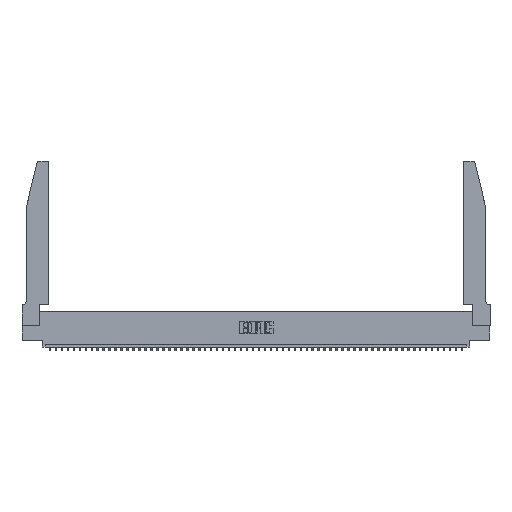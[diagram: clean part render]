
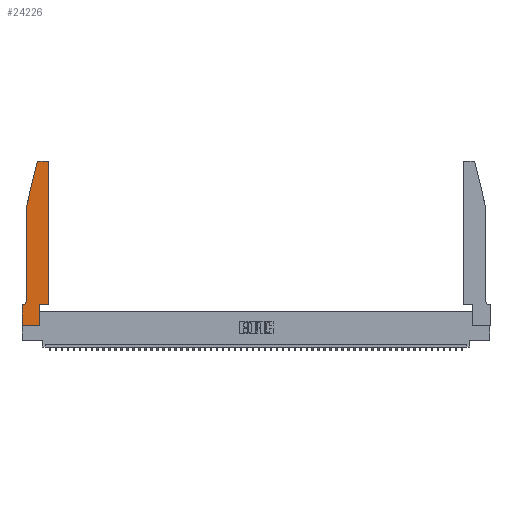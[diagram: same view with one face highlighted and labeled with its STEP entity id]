
A CAD part, top view. The second image highlights one B-rep face of the part: STEP entity #24226.
In plain terms, the highlighted planar face has unit normal (0, 0, 1).
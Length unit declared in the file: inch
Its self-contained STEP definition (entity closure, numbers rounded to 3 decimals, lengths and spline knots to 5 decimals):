
#601 = CARTESIAN_POINT ( 'NONE',  ( 0.284, 2.75, 0.37 ) ) ;
#662 = AXIS2_PLACEMENT_3D ( 'NONE', #33011, #7484, #36627 ) ;
#932 = VERTEX_POINT ( 'NONE', #28533 ) ;
#977 = ORIENTED_EDGE ( 'NONE', *, *, #35297, .T. ) ;
#1527 = CARTESIAN_POINT ( 'NONE',  ( 0.2865, 0.35, 0.37 ) ) ;
#1742 = LINE ( 'NONE', #27572, #7127 ) ;
#2084 = AXIS2_PLACEMENT_3D ( 'NONE', #19080, #23292, #15078 ) ;
#2785 = DIRECTION ( 'NONE',  ( 1., 0., 0. ) ) ;
#3431 = CARTESIAN_POINT ( 'NONE',  ( 0.25487, 2.72718, 0.37 ) ) ;
#3888 = CIRCLE ( 'NONE', #662, 0.03 ) ;
#4181 = AXIS2_PLACEMENT_3D ( 'NONE', #37291, #37455, #8630 ) ;
#4629 = VERTEX_POINT ( 'NONE', #11432 ) ;
#5304 = DIRECTION ( 'NONE',  ( 1., 0., 0. ) ) ;
#5510 = EDGE_CURVE ( 'NONE', #30403, #42698, #13013, .T. ) ;
#5828 = CARTESIAN_POINT ( 'NONE',  ( 0.4205, 2.72, 0.37 ) ) ;
#7127 = VECTOR ( 'NONE', #14575, 39.37008 ) ;
#7484 = DIRECTION ( 'NONE',  ( 0., 0., 1. ) ) ;
#7656 = EDGE_CURVE ( 'NONE', #35112, #29569, #52413, .T. ) ;
#7732 = ORIENTED_EDGE ( 'NONE', *, *, #39719, .T. ) ;
#8617 = DIRECTION ( 'NONE',  ( 0., -1., 0. ) ) ;
#8630 = DIRECTION ( 'NONE',  ( 1., 0., 0. ) ) ;
#9082 = CARTESIAN_POINT ( 'NONE',  ( 0., 0., 0.37 ) ) ;
#9317 = ORIENTED_EDGE ( 'NONE', *, *, #26377, .T. ) ;
#9449 = LINE ( 'NONE', #18105, #13400 ) ;
#11432 = CARTESIAN_POINT ( 'NONE',  ( 0.2865, 0., 0.37 ) ) ;
#11755 = EDGE_LOOP ( 'NONE', ( #43595, #7732, #24595, #18098, #31854, #32771, #25570, #9317, #977, #16857, #46579, #27250 ) ) ;
#11914 = DIRECTION ( 'NONE',  ( 0., 1., 0. ) ) ;
#13013 = LINE ( 'NONE', #13363, #38405 ) ;
#13363 = CARTESIAN_POINT ( 'NONE',  ( 0.4505, 0.35, 0.37 ) ) ;
#13400 = VECTOR ( 'NONE', #29985, 39.37008 ) ;
#14575 = DIRECTION ( 'NONE',  ( -1., 0., 0. ) ) ;
#14721 = LINE ( 'NONE', #31990, #43423 ) ;
#14738 = CARTESIAN_POINT ( 'NONE',  ( 0.0755, 2., 0.37 ) ) ;
#15078 = DIRECTION ( 'NONE',  ( -1., 0., 0. ) ) ;
#15636 = VERTEX_POINT ( 'NONE', #14738 ) ;
#16574 = VERTEX_POINT ( 'NONE', #3431 ) ;
#16857 = ORIENTED_EDGE ( 'NONE', *, *, #5510, .T. ) ;
#17246 = CIRCLE ( 'NONE', #2084, 0.07 ) ;
#18098 = ORIENTED_EDGE ( 'NONE', *, *, #46124, .T. ) ;
#18105 = CARTESIAN_POINT ( 'NONE',  ( 0.0755, 2., 0.37 ) ) ;
#18198 = EDGE_CURVE ( 'NONE', #16574, #15636, #14721, .T. ) ;
#18375 = CARTESIAN_POINT ( 'NONE',  ( 0.4505, 0.35, 0.37 ) ) ;
#19080 = CARTESIAN_POINT ( 'NONE',  ( 0.0055, 0.42, 0.37 ) ) ;
#21440 = LINE ( 'NONE', #1527, #44349 ) ;
#21649 = CARTESIAN_POINT ( 'NONE',  ( 0., 0., 0.37 ) ) ;
#21726 = AXIS2_PLACEMENT_3D ( 'NONE', #5828, #49214, #2785 ) ;
#22987 = EDGE_CURVE ( 'NONE', #46513, #932, #1742, .T. ) ;
#23178 = DIRECTION ( 'NONE',  ( -1., 0., 0. ) ) ;
#23292 = DIRECTION ( 'NONE',  ( 0., 0., -1. ) ) ;
#23734 = LINE ( 'NONE', #40146, #53000 ) ;
#23956 = CARTESIAN_POINT ( 'NONE',  ( 0.4205, 2.75, 0.37 ) ) ;
#24226 = ADVANCED_FACE ( 'NONE', ( #41902 ), #49429, .T. ) ;
#24595 = ORIENTED_EDGE ( 'NONE', *, *, #18198, .T. ) ;
#25435 = VERTEX_POINT ( 'NONE', #21649 ) ;
#25570 = ORIENTED_EDGE ( 'NONE', *, *, #50885, .T. ) ;
#26247 = VECTOR ( 'NONE', #5304, 39.37008 ) ;
#26377 = EDGE_CURVE ( 'NONE', #25435, #4629, #40033, .T. ) ;
#27250 = ORIENTED_EDGE ( 'NONE', *, *, #7656, .T. ) ;
#27572 = CARTESIAN_POINT ( 'NONE',  ( 0.0755, 0.35, 0.37 ) ) ;
#28533 = CARTESIAN_POINT ( 'NONE',  ( 0., 0.35, 0.37 ) ) ;
#29314 = CARTESIAN_POINT ( 'NONE',  ( 0.0755, 0.42, 0.37 ) ) ;
#29569 = VERTEX_POINT ( 'NONE', #23956 ) ;
#29985 = DIRECTION ( 'NONE',  ( 0., -1., 0. ) ) ;
#30403 = VERTEX_POINT ( 'NONE', #43623 ) ;
#31854 = ORIENTED_EDGE ( 'NONE', *, *, #50101, .T. ) ;
#31990 = CARTESIAN_POINT ( 'NONE',  ( 0.0755, 2., 0.37 ) ) ;
#32771 = ORIENTED_EDGE ( 'NONE', *, *, #22987, .T. ) ;
#33011 = CARTESIAN_POINT ( 'NONE',  ( 0.284, 2.72, 0.37 ) ) ;
#34296 = CARTESIAN_POINT ( 'NONE',  ( 0., 0., 0.37 ) ) ;
#34715 = VECTOR ( 'NONE', #11914, 39.37008 ) ;
#35112 = VERTEX_POINT ( 'NONE', #35997 ) ;
#35134 = DIRECTION ( 'NONE',  ( 0., 1., 0. ) ) ;
#35297 = EDGE_CURVE ( 'NONE', #4629, #30403, #21440, .T. ) ;
#35997 = CARTESIAN_POINT ( 'NONE',  ( 0.4505, 2.72, 0.37 ) ) ;
#36627 = DIRECTION ( 'NONE',  ( 1., 0., 0. ) ) ;
#37291 = CARTESIAN_POINT ( 'NONE',  ( 0., 0.35, 0.37 ) ) ;
#37455 = DIRECTION ( 'NONE',  ( 0., 0., 1. ) ) ;
#38405 = VECTOR ( 'NONE', #47194, 39.37008 ) ;
#39719 = EDGE_CURVE ( 'NONE', #44422, #16574, #3888, .T. ) ;
#40033 = LINE ( 'NONE', #34296, #26247 ) ;
#40146 = CARTESIAN_POINT ( 'NONE',  ( 0.2605, 2.75, 0.37 ) ) ;
#41902 = FACE_OUTER_BOUND ( 'NONE', #11755, .T. ) ;
#42698 = VERTEX_POINT ( 'NONE', #18375 ) ;
#42754 = EDGE_CURVE ( 'NONE', #29569, #44422, #23734, .T. ) ;
#42915 = EDGE_CURVE ( 'NONE', #42698, #35112, #45845, .T. ) ;
#43423 = VECTOR ( 'NONE', #52459, 39.37008 ) ;
#43595 = ORIENTED_EDGE ( 'NONE', *, *, #42754, .T. ) ;
#43623 = CARTESIAN_POINT ( 'NONE',  ( 0.2865, 0.35, 0.37 ) ) ;
#43921 = VECTOR ( 'NONE', #8617, 39.37008 ) ;
#44016 = CARTESIAN_POINT ( 'NONE',  ( 0.0055, 0.35, 0.37 ) ) ;
#44349 = VECTOR ( 'NONE', #35134, 39.37008 ) ;
#44354 = VERTEX_POINT ( 'NONE', #29314 ) ;
#44422 = VERTEX_POINT ( 'NONE', #601 ) ;
#44598 = LINE ( 'NONE', #9082, #43921 ) ;
#45845 = LINE ( 'NONE', #49567, #34715 ) ;
#46124 = EDGE_CURVE ( 'NONE', #15636, #44354, #9449, .T. ) ;
#46513 = VERTEX_POINT ( 'NONE', #44016 ) ;
#46579 = ORIENTED_EDGE ( 'NONE', *, *, #42915, .T. ) ;
#47194 = DIRECTION ( 'NONE',  ( 1., 0., 0. ) ) ;
#49214 = DIRECTION ( 'NONE',  ( 0., 0., 1. ) ) ;
#49429 = PLANE ( 'NONE',  #4181 ) ;
#49567 = CARTESIAN_POINT ( 'NONE',  ( 0.4505, 0.35, 0.37 ) ) ;
#50101 = EDGE_CURVE ( 'NONE', #44354, #46513, #17246, .T. ) ;
#50885 = EDGE_CURVE ( 'NONE', #932, #25435, #44598, .T. ) ;
#52413 = CIRCLE ( 'NONE', #21726, 0.03 ) ;
#52459 = DIRECTION ( 'NONE',  ( -0.239, -0.971, 0. ) ) ;
#53000 = VECTOR ( 'NONE', #23178, 39.37008 ) ;
